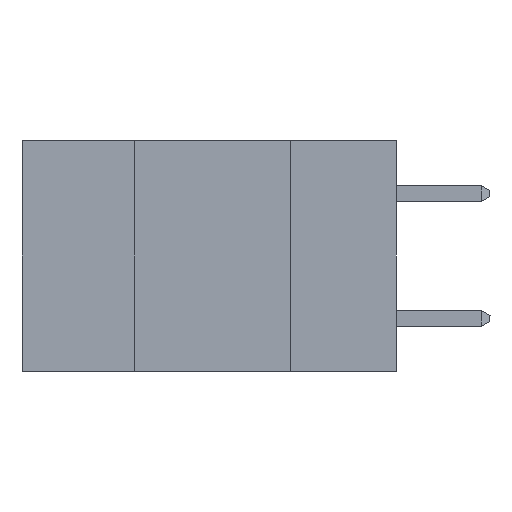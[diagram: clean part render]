
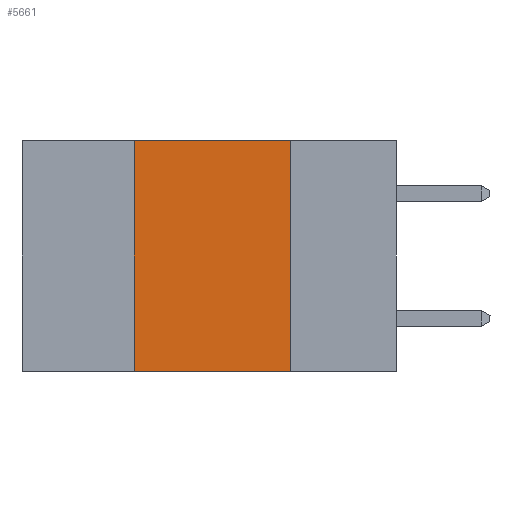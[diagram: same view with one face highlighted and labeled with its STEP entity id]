
A CAD part, left-side view. The second image highlights one B-rep face of the part: STEP entity #5661.
In plain terms, the highlighted planar face has unit normal (-1, 0, 0).
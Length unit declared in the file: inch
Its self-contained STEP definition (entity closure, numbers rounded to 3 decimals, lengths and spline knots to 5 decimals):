
#433 = DIRECTION ( 'NONE',  ( 0., 0., -1. ) ) ;
#458 = DIRECTION ( 'NONE',  ( 1., 0., 0. ) ) ;
#514 = PLANE ( 'NONE',  #6155 ) ;
#634 = DIRECTION ( 'NONE',  ( 0., -1., 0. ) ) ;
#715 = CARTESIAN_POINT ( 'NONE',  ( 0., 0.6, 0. ) ) ;
#777 = CARTESIAN_POINT ( 'NONE',  ( 0., 0.6, 0. ) ) ;
#1461 = EDGE_CURVE ( 'NONE', #10099, #4221, #4377, .T. ) ;
#1535 = ORIENTED_EDGE ( 'NONE', *, *, #1461, .F. ) ;
#1563 = CARTESIAN_POINT ( 'NONE',  ( 0., 0.17, 0. ) ) ;
#2178 = CARTESIAN_POINT ( 'NONE',  ( 0., 0.42, 0. ) ) ;
#2301 = EDGE_CURVE ( 'NONE', #4221, #2971, #11583, .T. ) ;
#2971 = VERTEX_POINT ( 'NONE', #9989 ) ;
#3991 = VECTOR ( 'NONE', #634, 39.37008 ) ;
#4221 = VERTEX_POINT ( 'NONE', #1563 ) ;
#4377 = LINE ( 'NONE', #715, #3991 ) ;
#4531 = CARTESIAN_POINT ( 'NONE',  ( 0., 0.42, -0.37 ) ) ;
#4606 = DIRECTION ( 'NONE',  ( 0., 0., 1. ) ) ;
#4896 = LINE ( 'NONE', #9696, #7609 ) ;
#5661 = ADVANCED_FACE ( 'NONE', ( #9676 ), #514, .F. ) ;
#6155 = AXIS2_PLACEMENT_3D ( 'NONE', #777, #458, #433 ) ;
#7609 = VECTOR ( 'NONE', #9723, 39.37008 ) ;
#7757 = LINE ( 'NONE', #4531, #10382 ) ;
#8293 = ORIENTED_EDGE ( 'NONE', *, *, #14634, .F. ) ;
#9676 = FACE_OUTER_BOUND ( 'NONE', #14848, .T. ) ;
#9696 = CARTESIAN_POINT ( 'NONE',  ( 0., 0.6, -0.37 ) ) ;
#9723 = DIRECTION ( 'NONE',  ( 0., -1., 0. ) ) ;
#9989 = CARTESIAN_POINT ( 'NONE',  ( 0., 0.17, -0.37 ) ) ;
#10099 = VERTEX_POINT ( 'NONE', #2178 ) ;
#10382 = VECTOR ( 'NONE', #4606, 39.37008 ) ;
#11140 = CARTESIAN_POINT ( 'NONE',  ( 0., 0.42, -0.37 ) ) ;
#11213 = ORIENTED_EDGE ( 'NONE', *, *, #13972, .T. ) ;
#11254 = VECTOR ( 'NONE', #14754, 39.37008 ) ;
#11583 = LINE ( 'NONE', #14790, #11254 ) ;
#11914 = VERTEX_POINT ( 'NONE', #11140 ) ;
#13364 = ORIENTED_EDGE ( 'NONE', *, *, #2301, .F. ) ;
#13972 = EDGE_CURVE ( 'NONE', #11914, #2971, #4896, .T. ) ;
#14634 = EDGE_CURVE ( 'NONE', #11914, #10099, #7757, .T. ) ;
#14754 = DIRECTION ( 'NONE',  ( 0., 0., -1. ) ) ;
#14790 = CARTESIAN_POINT ( 'NONE',  ( 0., 0.17, -0.37 ) ) ;
#14848 = EDGE_LOOP ( 'NONE', ( #13364, #1535, #8293, #11213 ) ) ;
